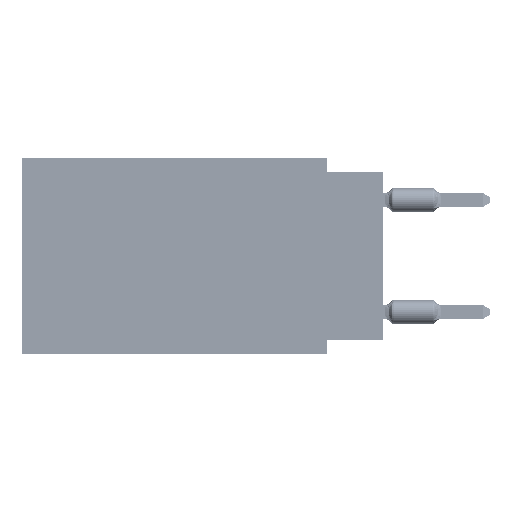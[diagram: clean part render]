
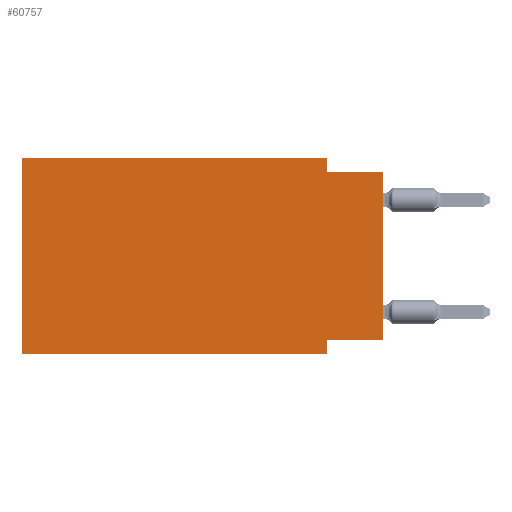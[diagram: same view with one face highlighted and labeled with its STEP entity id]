
A CAD part, left-side view. The second image highlights one B-rep face of the part: STEP entity #60757.
In plain terms, the highlighted planar face has unit normal (-1, 0, 0).
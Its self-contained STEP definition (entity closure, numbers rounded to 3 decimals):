
#1178 = VERTEX_POINT ( 'NONE', #83289 ) ;
#1812 = CARTESIAN_POINT ( 'NONE',  ( 0., 16.383, -8.89 ) ) ;
#3960 = DIRECTION ( 'NONE',  ( 0., 0., 1. ) ) ;
#5170 = CARTESIAN_POINT ( 'NONE',  ( 0., 2.54, -0.635 ) ) ;
#7749 = EDGE_CURVE ( 'NONE', #1178, #24324, #46569, .T. ) ;
#8435 = CARTESIAN_POINT ( 'NONE',  ( 0., 0., -8.255 ) ) ;
#9765 = CARTESIAN_POINT ( 'NONE',  ( 0., 2.54, 0. ) ) ;
#13089 = DIRECTION ( 'NONE',  ( 0., 0., 1. ) ) ;
#13561 = LINE ( 'NONE', #64978, #44378 ) ;
#16876 = DIRECTION ( 'NONE',  ( 1., 0., 0. ) ) ;
#19379 = EDGE_CURVE ( 'NONE', #71307, #1178, #37148, .T. ) ;
#19979 = EDGE_CURVE ( 'NONE', #48266, #106259, #32714, .T. ) ;
#20389 = CARTESIAN_POINT ( 'NONE',  ( 0., 0., 0. ) ) ;
#22628 = ORIENTED_EDGE ( 'NONE', *, *, #78673, .F. ) ;
#23151 = ORIENTED_EDGE ( 'NONE', *, *, #95317, .T. ) ;
#24324 = VERTEX_POINT ( 'NONE', #71391 ) ;
#28161 = ORIENTED_EDGE ( 'NONE', *, *, #64176, .T. ) ;
#30220 = CARTESIAN_POINT ( 'NONE',  ( 0., 0., -0.635 ) ) ;
#32714 = LINE ( 'NONE', #66123, #79162 ) ;
#34619 = DIRECTION ( 'NONE',  ( 0., -1., 0. ) ) ;
#35629 = CARTESIAN_POINT ( 'NONE',  ( 0., 0., -0.635 ) ) ;
#36541 = VECTOR ( 'NONE', #60266, 1000. ) ;
#37148 = LINE ( 'NONE', #70565, #79075 ) ;
#38146 = DIRECTION ( 'NONE',  ( 0., -1., 0. ) ) ;
#43070 = FACE_OUTER_BOUND ( 'NONE', #66693, .T. ) ;
#43082 = VERTEX_POINT ( 'NONE', #5170 ) ;
#44220 = ORIENTED_EDGE ( 'NONE', *, *, #19379, .F. ) ;
#44378 = VECTOR ( 'NONE', #38146, 1000. ) ;
#46569 = LINE ( 'NONE', #79990, #53981 ) ;
#48266 = VERTEX_POINT ( 'NONE', #77519 ) ;
#50210 = DIRECTION ( 'NONE',  ( 0., 0., -1. ) ) ;
#51058 = DIRECTION ( 'NONE',  ( 0., 1., 0. ) ) ;
#52857 = CARTESIAN_POINT ( 'NONE',  ( 0., 2.54, -8.89 ) ) ;
#53981 = VECTOR ( 'NONE', #34619, 1000. ) ;
#56793 = VECTOR ( 'NONE', #51058, 1000. ) ;
#57540 = ORIENTED_EDGE ( 'NONE', *, *, #102278, .F. ) ;
#58439 = PLANE ( 'NONE',  #61378 ) ;
#60266 = DIRECTION ( 'NONE',  ( 0., -1., 0. ) ) ;
#60757 = ADVANCED_FACE ( 'NONE', ( #43070 ), #58439, .F. ) ;
#61378 = AXIS2_PLACEMENT_3D ( 'NONE', #91829, #16876, #50210 ) ;
#64176 = EDGE_CURVE ( 'NONE', #94144, #101570, #78928, .T. ) ;
#64480 = ORIENTED_EDGE ( 'NONE', *, *, #7749, .F. ) ;
#64978 = CARTESIAN_POINT ( 'NONE',  ( 0., 16.383, -8.89 ) ) ;
#66123 = CARTESIAN_POINT ( 'NONE',  ( 0., 2.54, -8.89 ) ) ;
#66693 = EDGE_LOOP ( 'NONE', ( #28161, #22628, #57540, #64480, #44220, #23151, #105038, #95113 ) ) ;
#70565 = CARTESIAN_POINT ( 'NONE',  ( 0., 16.383, 0. ) ) ;
#71307 = VERTEX_POINT ( 'NONE', #1812 ) ;
#71391 = CARTESIAN_POINT ( 'NONE',  ( 0., 2.54, 0. ) ) ;
#74100 = VECTOR ( 'NONE', #3960, 1000. ) ;
#75929 = VECTOR ( 'NONE', #76546, 1000. ) ;
#76546 = DIRECTION ( 'NONE',  ( 0., 0., -1. ) ) ;
#77519 = CARTESIAN_POINT ( 'NONE',  ( 0., 2.54, -8.255 ) ) ;
#78673 = EDGE_CURVE ( 'NONE', #43082, #101570, #93653, .T. ) ;
#78928 = LINE ( 'NONE', #20389, #74100 ) ;
#79075 = VECTOR ( 'NONE', #13089, 1000. ) ;
#79162 = VECTOR ( 'NONE', #99475, 1000. ) ;
#79990 = CARTESIAN_POINT ( 'NONE',  ( 0., 16.383, 0. ) ) ;
#83289 = CARTESIAN_POINT ( 'NONE',  ( 0., 16.383, 0. ) ) ;
#84753 = LINE ( 'NONE', #9765, #75929 ) ;
#86295 = CARTESIAN_POINT ( 'NONE',  ( 0., 0., -8.255 ) ) ;
#91829 = CARTESIAN_POINT ( 'NONE',  ( 0., 16.383, 0. ) ) ;
#93653 = LINE ( 'NONE', #35629, #36541 ) ;
#94144 = VERTEX_POINT ( 'NONE', #86295 ) ;
#95113 = ORIENTED_EDGE ( 'NONE', *, *, #104799, .F. ) ;
#95317 = EDGE_CURVE ( 'NONE', #71307, #106259, #13561, .T. ) ;
#99475 = DIRECTION ( 'NONE',  ( 0., 0., -1. ) ) ;
#100886 = LINE ( 'NONE', #8435, #56793 ) ;
#101570 = VERTEX_POINT ( 'NONE', #30220 ) ;
#102278 = EDGE_CURVE ( 'NONE', #24324, #43082, #84753, .T. ) ;
#104799 = EDGE_CURVE ( 'NONE', #94144, #48266, #100886, .T. ) ;
#105038 = ORIENTED_EDGE ( 'NONE', *, *, #19979, .F. ) ;
#106259 = VERTEX_POINT ( 'NONE', #52857 ) ;
